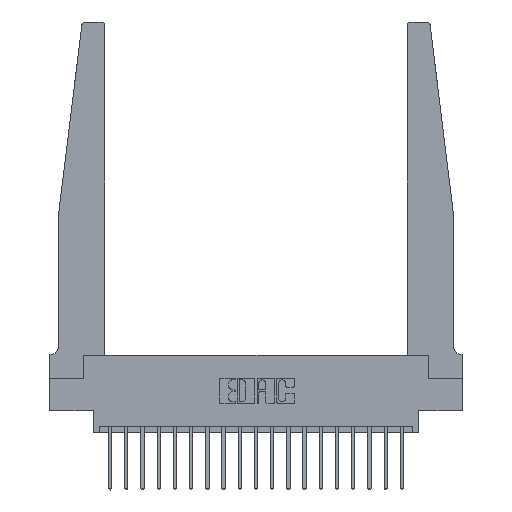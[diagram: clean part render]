
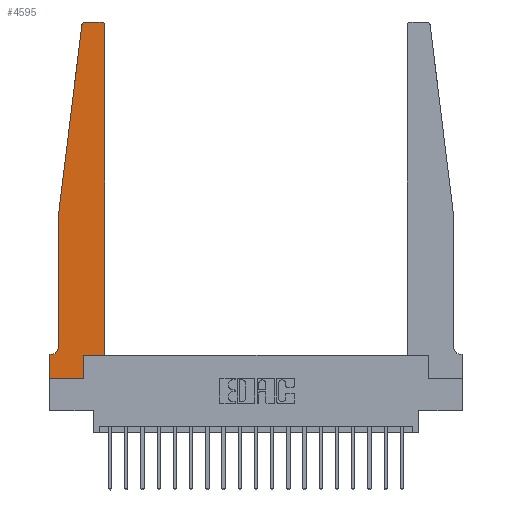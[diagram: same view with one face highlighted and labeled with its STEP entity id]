
A CAD part, top view. The second image highlights one B-rep face of the part: STEP entity #4595.
In plain terms, the highlighted planar face has unit normal (0, 0, 1).
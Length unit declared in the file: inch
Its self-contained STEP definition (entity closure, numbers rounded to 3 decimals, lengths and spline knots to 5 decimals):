
#262 = VERTEX_POINT ( 'NONE', #16130 ) ;
#713 = VECTOR ( 'NONE', #17365, 39.37008 ) ;
#739 = DIRECTION ( 'NONE',  ( 0., -1., 0. ) ) ;
#846 = CARTESIAN_POINT ( 'NONE',  ( 0.27653, 2.75, 0.37 ) ) ;
#1045 = VECTOR ( 'NONE', #12577, 39.37008 ) ;
#1077 = VECTOR ( 'NONE', #8836, 39.37008 ) ;
#1323 = DIRECTION ( 'NONE',  ( -1., 0., 0. ) ) ;
#1324 = CARTESIAN_POINT ( 'NONE',  ( 0., 0.1875, 0.37 ) ) ;
#1360 = EDGE_CURVE ( 'NONE', #13394, #16473, #3205, .T. ) ;
#1645 = CARTESIAN_POINT ( 'NONE',  ( 0.015, 0.1875, 0.37 ) ) ;
#1681 = EDGE_CURVE ( 'NONE', #13208, #262, #14556, .T. ) ;
#1737 = DIRECTION ( 'NONE',  ( 1., 0., 0. ) ) ;
#2220 = EDGE_CURVE ( 'NONE', #17504, #6291, #5164, .T. ) ;
#2300 = VERTEX_POINT ( 'NONE', #16760 ) ;
#2534 = CARTESIAN_POINT ( 'NONE',  ( 0.395, 2.72, 0.37 ) ) ;
#2627 = DIRECTION ( 'NONE',  ( 0., 0., 1. ) ) ;
#2961 = CARTESIAN_POINT ( 'NONE',  ( 0.27653, 2.72, 0.37 ) ) ;
#3159 = EDGE_CURVE ( 'NONE', #17893, #8087, #10350, .T. ) ;
#3205 = CIRCLE ( 'NONE', #14565, 0.03 ) ;
#3352 = LINE ( 'NONE', #16206, #16948 ) ;
#3482 = EDGE_CURVE ( 'NONE', #6435, #2300, #8613, .T. ) ;
#3573 = ORIENTED_EDGE ( 'NONE', *, *, #3159, .T. ) ;
#3850 = CARTESIAN_POINT ( 'NONE',  ( 0., 0., 0.37 ) ) ;
#3876 = CIRCLE ( 'NONE', #15012, 0.05 ) ;
#4142 = DIRECTION ( 'NONE',  ( 1., 0., 0. ) ) ;
#4180 = CARTESIAN_POINT ( 'NONE',  ( 0.065, 1.25, 0.37 ) ) ;
#4268 = ORIENTED_EDGE ( 'NONE', *, *, #16034, .T. ) ;
#4568 = DIRECTION ( 'NONE',  ( 1., 0., 0. ) ) ;
#4595 = ADVANCED_FACE ( 'NONE', ( #8468 ), #12150, .T. ) ;
#4631 = VECTOR ( 'NONE', #5236, 39.37008 ) ;
#4928 = VERTEX_POINT ( 'NONE', #18646 ) ;
#5164 = LINE ( 'NONE', #13382, #17247 ) ;
#5236 = DIRECTION ( 'NONE',  ( -1., 0., 0. ) ) ;
#5281 = CARTESIAN_POINT ( 'NONE',  ( 0., 0., 0.37 ) ) ;
#6180 = VECTOR ( 'NONE', #8609, 39.37008 ) ;
#6291 = VERTEX_POINT ( 'NONE', #14677 ) ;
#6435 = VERTEX_POINT ( 'NONE', #16614 ) ;
#6893 = DIRECTION ( 'NONE',  ( 1., 0., 0. ) ) ;
#7701 = CARTESIAN_POINT ( 'NONE',  ( 0.2605, 0.18, 0.37 ) ) ;
#7765 = EDGE_CURVE ( 'NONE', #17225, #13208, #9092, .T. ) ;
#8087 = VERTEX_POINT ( 'NONE', #16951 ) ;
#8390 = DIRECTION ( 'NONE',  ( 0., 1., 0. ) ) ;
#8468 = FACE_OUTER_BOUND ( 'NONE', #19286, .T. ) ;
#8609 = DIRECTION ( 'NONE',  ( 0., -1., 0. ) ) ;
#8613 = CIRCLE ( 'NONE', #10419, 0.03 ) ;
#8833 = LINE ( 'NONE', #5281, #12511 ) ;
#8836 = DIRECTION ( 'NONE',  ( -1., 0., 0. ) ) ;
#9092 = LINE ( 'NONE', #16268, #4631 ) ;
#9368 = VECTOR ( 'NONE', #1737, 39.37008 ) ;
#9523 = LINE ( 'NONE', #19798, #1077 ) ;
#10350 = LINE ( 'NONE', #17475, #9368 ) ;
#10419 = AXIS2_PLACEMENT_3D ( 'NONE', #2534, #13594, #4142 ) ;
#10822 = DIRECTION ( 'NONE',  ( 0., 0., -1. ) ) ;
#11424 = ORIENTED_EDGE ( 'NONE', *, *, #1681, .T. ) ;
#11588 = EDGE_CURVE ( 'NONE', #4928, #17893, #3352, .T. ) ;
#12084 = CARTESIAN_POINT ( 'NONE',  ( 0., 0.1875, 0.37 ) ) ;
#12150 = PLANE ( 'NONE',  #14468 ) ;
#12225 = EDGE_CURVE ( 'NONE', #262, #4928, #8833, .T. ) ;
#12443 = CARTESIAN_POINT ( 'NONE',  ( 0.065, 1.25, 0.37 ) ) ;
#12511 = VECTOR ( 'NONE', #6893, 39.37008 ) ;
#12577 = DIRECTION ( 'NONE',  ( -0.122, -0.992, 0. ) ) ;
#12649 = CARTESIAN_POINT ( 'NONE',  ( 0.425, 0.18, 0.37 ) ) ;
#13127 = ORIENTED_EDGE ( 'NONE', *, *, #2220, .T. ) ;
#13208 = VERTEX_POINT ( 'NONE', #1324 ) ;
#13326 = LINE ( 'NONE', #12649, #713 ) ;
#13382 = CARTESIAN_POINT ( 'NONE',  ( 0.065, 1.25, 0.37 ) ) ;
#13394 = VERTEX_POINT ( 'NONE', #846 ) ;
#13413 = EDGE_CURVE ( 'NONE', #2300, #13394, #9523, .T. ) ;
#13594 = DIRECTION ( 'NONE',  ( 0., 0., 1. ) ) ;
#13624 = LINE ( 'NONE', #12443, #1045 ) ;
#13687 = DIRECTION ( 'NONE',  ( 1., 0., 0. ) ) ;
#13754 = ORIENTED_EDGE ( 'NONE', *, *, #13413, .T. ) ;
#13849 = ORIENTED_EDGE ( 'NONE', *, *, #7765, .T. ) ;
#14020 = DIRECTION ( 'NONE',  ( 0., 0., 1. ) ) ;
#14301 = EDGE_CURVE ( 'NONE', #16473, #17504, #13624, .T. ) ;
#14468 = AXIS2_PLACEMENT_3D ( 'NONE', #12084, #2627, #13687 ) ;
#14556 = LINE ( 'NONE', #3850, #6180 ) ;
#14565 = AXIS2_PLACEMENT_3D ( 'NONE', #2961, #14020, #4568 ) ;
#14677 = CARTESIAN_POINT ( 'NONE',  ( 0.065, 0.2375, 0.37 ) ) ;
#15012 = AXIS2_PLACEMENT_3D ( 'NONE', #20189, #10822, #1323 ) ;
#15430 = ORIENTED_EDGE ( 'NONE', *, *, #14301, .T. ) ;
#16034 = EDGE_CURVE ( 'NONE', #8087, #6435, #13326, .T. ) ;
#16130 = CARTESIAN_POINT ( 'NONE',  ( 0., 0., 0.37 ) ) ;
#16206 = CARTESIAN_POINT ( 'NONE',  ( 0.2605, 0.18, 0.37 ) ) ;
#16268 = CARTESIAN_POINT ( 'NONE',  ( 0.065, 0.1875, 0.37 ) ) ;
#16473 = VERTEX_POINT ( 'NONE', #19943 ) ;
#16550 = ORIENTED_EDGE ( 'NONE', *, *, #17093, .T. ) ;
#16614 = CARTESIAN_POINT ( 'NONE',  ( 0.425, 2.72, 0.37 ) ) ;
#16760 = CARTESIAN_POINT ( 'NONE',  ( 0.395, 2.75, 0.37 ) ) ;
#16886 = ORIENTED_EDGE ( 'NONE', *, *, #12225, .T. ) ;
#16948 = VECTOR ( 'NONE', #8390, 39.37008 ) ;
#16951 = CARTESIAN_POINT ( 'NONE',  ( 0.425, 0.18, 0.37 ) ) ;
#17093 = EDGE_CURVE ( 'NONE', #6291, #17225, #3876, .T. ) ;
#17225 = VERTEX_POINT ( 'NONE', #1645 ) ;
#17247 = VECTOR ( 'NONE', #739, 39.37008 ) ;
#17365 = DIRECTION ( 'NONE',  ( 0., 1., 0. ) ) ;
#17475 = CARTESIAN_POINT ( 'NONE',  ( 0.425, 0.18, 0.37 ) ) ;
#17504 = VERTEX_POINT ( 'NONE', #4180 ) ;
#17832 = ORIENTED_EDGE ( 'NONE', *, *, #11588, .T. ) ;
#17893 = VERTEX_POINT ( 'NONE', #7701 ) ;
#18646 = CARTESIAN_POINT ( 'NONE',  ( 0.2605, 0., 0.37 ) ) ;
#19148 = ORIENTED_EDGE ( 'NONE', *, *, #3482, .T. ) ;
#19286 = EDGE_LOOP ( 'NONE', ( #13754, #19898, #15430, #13127, #16550, #13849, #11424, #16886, #17832, #3573, #4268, #19148 ) ) ;
#19798 = CARTESIAN_POINT ( 'NONE',  ( 0.25, 2.75, 0.37 ) ) ;
#19898 = ORIENTED_EDGE ( 'NONE', *, *, #1360, .T. ) ;
#19943 = CARTESIAN_POINT ( 'NONE',  ( 0.24675, 2.72367, 0.37 ) ) ;
#20189 = CARTESIAN_POINT ( 'NONE',  ( 0.015, 0.2375, 0.37 ) ) ;
